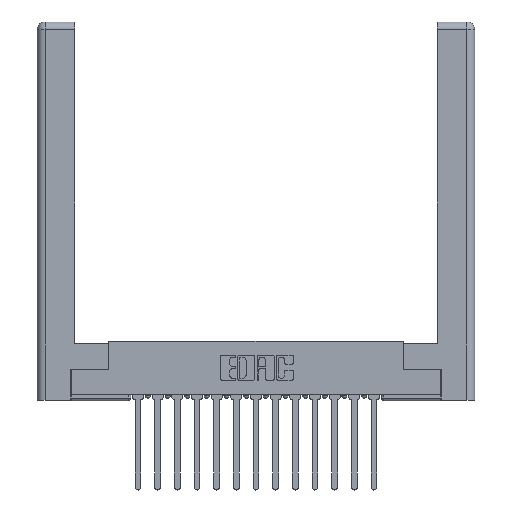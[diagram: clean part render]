
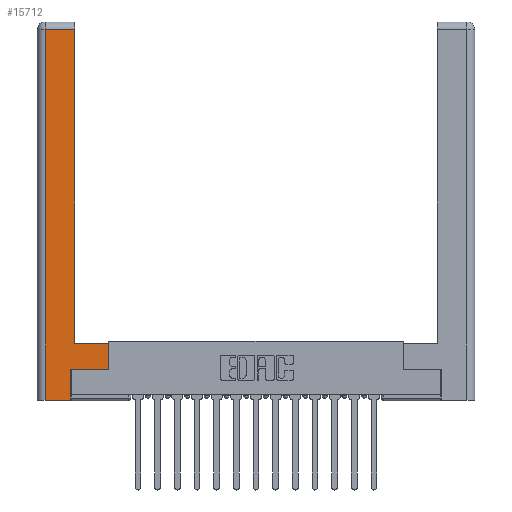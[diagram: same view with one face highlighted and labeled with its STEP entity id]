
A CAD part, top view. The second image highlights one B-rep face of the part: STEP entity #15712.
In plain terms, the highlighted planar face has unit normal (0, 0, 1).
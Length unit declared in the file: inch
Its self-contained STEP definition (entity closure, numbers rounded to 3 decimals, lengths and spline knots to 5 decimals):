
#357 = CARTESIAN_POINT ( 'NONE',  ( 0.565, 0.45, 0. ) ) ;
#634 = VERTEX_POINT ( 'NONE', #8153 ) ;
#721 = DIRECTION ( 'NONE',  ( -1., 0., 0. ) ) ;
#841 = LINE ( 'NONE', #6202, #3544 ) ;
#921 = DIRECTION ( 'NONE',  ( 0., 1., 0. ) ) ;
#1177 = PLANE ( 'NONE',  #7761 ) ;
#1213 = CARTESIAN_POINT ( 'NONE',  ( 0.565, 0.245, 0. ) ) ;
#1252 = CARTESIAN_POINT ( 'NONE',  ( 0.265, 0.245, 0. ) ) ;
#2073 = VERTEX_POINT ( 'NONE', #357 ) ;
#2323 = LINE ( 'NONE', #12919, #10981 ) ;
#2846 = VERTEX_POINT ( 'NONE', #1252 ) ;
#3024 = DIRECTION ( 'NONE',  ( 0., -1., 0. ) ) ;
#3544 = VECTOR ( 'NONE', #11536, 39.37008 ) ;
#3658 = EDGE_CURVE ( 'NONE', #2846, #15225, #8682, .T. ) ;
#3802 = CARTESIAN_POINT ( 'NONE',  ( 0.295, 3., 0. ) ) ;
#3809 = CARTESIAN_POINT ( 'NONE',  ( 0., 0., 0. ) ) ;
#3833 = VECTOR ( 'NONE', #3024, 39.37008 ) ;
#4761 = VERTEX_POINT ( 'NONE', #6054 ) ;
#4795 = CARTESIAN_POINT ( 'NONE',  ( 0.0615, 2.94, 0. ) ) ;
#4804 = CARTESIAN_POINT ( 'NONE',  ( 0.565, 0.245, 0. ) ) ;
#5346 = VERTEX_POINT ( 'NONE', #15733 ) ;
#5480 = CARTESIAN_POINT ( 'NONE',  ( 0.0615, 0., 0. ) ) ;
#5559 = VERTEX_POINT ( 'NONE', #8044 ) ;
#5804 = VECTOR ( 'NONE', #721, 39.37008 ) ;
#6002 = ORIENTED_EDGE ( 'NONE', *, *, #3658, .T. ) ;
#6054 = CARTESIAN_POINT ( 'NONE',  ( 0.0615, 0., 0. ) ) ;
#6202 = CARTESIAN_POINT ( 'NONE',  ( 0.265, 0.245, 0. ) ) ;
#6658 = CARTESIAN_POINT ( 'NONE',  ( 0.0615, 2.94, 0. ) ) ;
#7523 = DIRECTION ( 'NONE',  ( -1., 0., 0. ) ) ;
#7549 = EDGE_LOOP ( 'NONE', ( #8883, #9499, #12430, #10663, #17164, #6002, #8204, #17087 ) ) ;
#7683 = EDGE_CURVE ( 'NONE', #5346, #2846, #841, .T. ) ;
#7761 = AXIS2_PLACEMENT_3D ( 'NONE', #3809, #10298, #10554 ) ;
#7849 = EDGE_CURVE ( 'NONE', #8554, #4761, #9687, .T. ) ;
#8044 = CARTESIAN_POINT ( 'NONE',  ( 0.295, 0.45, 0. ) ) ;
#8153 = CARTESIAN_POINT ( 'NONE',  ( 0.295, 2.94, 0. ) ) ;
#8204 = ORIENTED_EDGE ( 'NONE', *, *, #11628, .T. ) ;
#8554 = VERTEX_POINT ( 'NONE', #6658 ) ;
#8682 = LINE ( 'NONE', #1213, #14950 ) ;
#8883 = ORIENTED_EDGE ( 'NONE', *, *, #9478, .T. ) ;
#8914 = EDGE_CURVE ( 'NONE', #634, #8554, #11539, .T. ) ;
#8975 = VECTOR ( 'NONE', #11768, 39.37008 ) ;
#9278 = DIRECTION ( 'NONE',  ( 1., 0., 0. ) ) ;
#9416 = DIRECTION ( 'NONE',  ( 1., 0., 0. ) ) ;
#9478 = EDGE_CURVE ( 'NONE', #5559, #634, #16056, .T. ) ;
#9499 = ORIENTED_EDGE ( 'NONE', *, *, #8914, .T. ) ;
#9687 = LINE ( 'NONE', #5480, #3833 ) ;
#10298 = DIRECTION ( 'NONE',  ( 0., 0., -1. ) ) ;
#10554 = DIRECTION ( 'NONE',  ( -1., 0., 0. ) ) ;
#10663 = ORIENTED_EDGE ( 'NONE', *, *, #12966, .T. ) ;
#10981 = VECTOR ( 'NONE', #921, 39.37008 ) ;
#11018 = VECTOR ( 'NONE', #9416, 39.37008 ) ;
#11536 = DIRECTION ( 'NONE',  ( 0., 1., 0. ) ) ;
#11539 = LINE ( 'NONE', #4795, #12866 ) ;
#11628 = EDGE_CURVE ( 'NONE', #15225, #2073, #2323, .T. ) ;
#11768 = DIRECTION ( 'NONE',  ( 0., 1., 0. ) ) ;
#12430 = ORIENTED_EDGE ( 'NONE', *, *, #7849, .T. ) ;
#12866 = VECTOR ( 'NONE', #7523, 39.37008 ) ;
#12919 = CARTESIAN_POINT ( 'NONE',  ( 0.565, 0.45, 0. ) ) ;
#12966 = EDGE_CURVE ( 'NONE', #4761, #5346, #13619, .T. ) ;
#13619 = LINE ( 'NONE', #17307, #11018 ) ;
#13958 = LINE ( 'NONE', #16587, #5804 ) ;
#14950 = VECTOR ( 'NONE', #9278, 39.37008 ) ;
#15225 = VERTEX_POINT ( 'NONE', #4804 ) ;
#15712 = ADVANCED_FACE ( 'NONE', ( #17045 ), #1177, .F. ) ;
#15733 = CARTESIAN_POINT ( 'NONE',  ( 0.265, 0., 0. ) ) ;
#16047 = EDGE_CURVE ( 'NONE', #2073, #5559, #13958, .T. ) ;
#16056 = LINE ( 'NONE', #3802, #8975 ) ;
#16587 = CARTESIAN_POINT ( 'NONE',  ( 0.295, 0.45, 0. ) ) ;
#17045 = FACE_OUTER_BOUND ( 'NONE', #7549, .T. ) ;
#17087 = ORIENTED_EDGE ( 'NONE', *, *, #16047, .T. ) ;
#17164 = ORIENTED_EDGE ( 'NONE', *, *, #7683, .T. ) ;
#17307 = CARTESIAN_POINT ( 'NONE',  ( 0.265, 0., 0. ) ) ;
